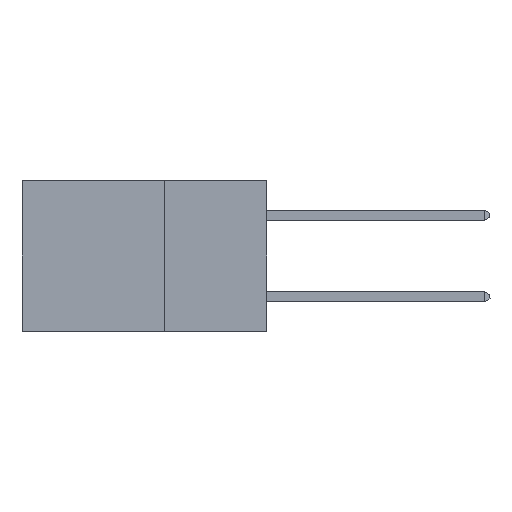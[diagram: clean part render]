
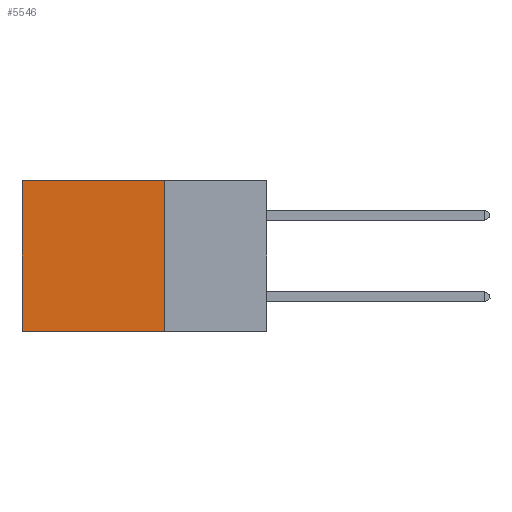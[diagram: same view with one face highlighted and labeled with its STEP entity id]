
A CAD part, left-side view. The second image highlights one B-rep face of the part: STEP entity #5546.
In plain terms, the highlighted planar face has unit normal (-1, 0, 0).
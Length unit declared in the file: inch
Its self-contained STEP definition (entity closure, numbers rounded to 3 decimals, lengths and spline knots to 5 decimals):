
#639 = VERTEX_POINT ( 'NONE', #7737 ) ;
#961 = EDGE_CURVE ( 'NONE', #11707, #11774, #9280, .T. ) ;
#1041 = EDGE_CURVE ( 'NONE', #639, #5678, #13495, .T. ) ;
#2712 = FACE_OUTER_BOUND ( 'NONE', #15914, .T. ) ;
#2867 = CARTESIAN_POINT ( 'NONE',  ( 0.2875, 0.25, 0. ) ) ;
#3849 = LINE ( 'NONE', #2867, #14471 ) ;
#3880 = VECTOR ( 'NONE', #10793, 39.37008 ) ;
#4353 = AXIS2_PLACEMENT_3D ( 'NONE', #16531, #12759, #9323 ) ;
#5546 = ADVANCED_FACE ( 'NONE', ( #2712 ), #12488, .F. ) ;
#5576 = DIRECTION ( 'NONE',  ( 0., 1., 0. ) ) ;
#5678 = VERTEX_POINT ( 'NONE', #16340 ) ;
#6021 = ORIENTED_EDGE ( 'NONE', *, *, #961, .F. ) ;
#6080 = EDGE_CURVE ( 'NONE', #5678, #11774, #10922, .T. ) ;
#7018 = ORIENTED_EDGE ( 'NONE', *, *, #1041, .T. ) ;
#7132 = CARTESIAN_POINT ( 'NONE',  ( 0.2875, 0.6, -0.37 ) ) ;
#7502 = CARTESIAN_POINT ( 'NONE',  ( 0.2875, 0.25, 0. ) ) ;
#7737 = CARTESIAN_POINT ( 'NONE',  ( 0.2875, 0.25, 0. ) ) ;
#7894 = VECTOR ( 'NONE', #16187, 39.37008 ) ;
#8125 = CARTESIAN_POINT ( 'NONE',  ( 0.2875, 0.25, -0.37 ) ) ;
#8756 = CARTESIAN_POINT ( 'NONE',  ( 0.2875, 0.6, 0. ) ) ;
#8891 = ORIENTED_EDGE ( 'NONE', *, *, #13682, .F. ) ;
#9280 = LINE ( 'NONE', #13265, #9477 ) ;
#9323 = DIRECTION ( 'NONE',  ( 0., 0., -1. ) ) ;
#9477 = VECTOR ( 'NONE', #5576, 39.37008 ) ;
#10450 = ORIENTED_EDGE ( 'NONE', *, *, #6080, .T. ) ;
#10793 = DIRECTION ( 'NONE',  ( 0., 0., -1. ) ) ;
#10922 = LINE ( 'NONE', #8756, #3880 ) ;
#11707 = VERTEX_POINT ( 'NONE', #8125 ) ;
#11750 = DIRECTION ( 'NONE',  ( 0., 0., -1. ) ) ;
#11774 = VERTEX_POINT ( 'NONE', #7132 ) ;
#12488 = PLANE ( 'NONE',  #4353 ) ;
#12759 = DIRECTION ( 'NONE',  ( 1., 0., 0. ) ) ;
#13265 = CARTESIAN_POINT ( 'NONE',  ( 0.2875, 0.25, -0.37 ) ) ;
#13495 = LINE ( 'NONE', #7502, #7894 ) ;
#13682 = EDGE_CURVE ( 'NONE', #639, #11707, #3849, .T. ) ;
#14471 = VECTOR ( 'NONE', #11750, 39.37008 ) ;
#15914 = EDGE_LOOP ( 'NONE', ( #10450, #6021, #8891, #7018 ) ) ;
#16187 = DIRECTION ( 'NONE',  ( 0., 1., 0. ) ) ;
#16340 = CARTESIAN_POINT ( 'NONE',  ( 0.2875, 0.6, 0. ) ) ;
#16531 = CARTESIAN_POINT ( 'NONE',  ( 0.2875, 0.25, 0. ) ) ;
